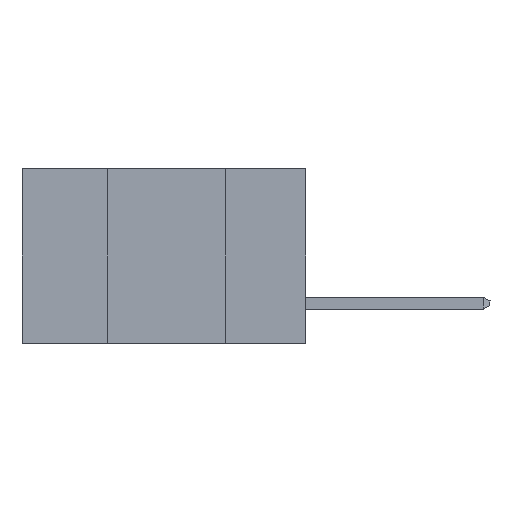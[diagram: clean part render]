
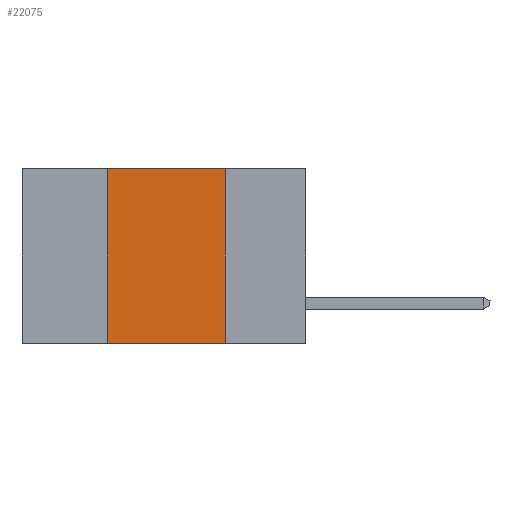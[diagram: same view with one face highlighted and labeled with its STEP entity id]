
A CAD part, left-side view. The second image highlights one B-rep face of the part: STEP entity #22075.
In plain terms, the highlighted planar face has unit normal (-1, 0, 0).
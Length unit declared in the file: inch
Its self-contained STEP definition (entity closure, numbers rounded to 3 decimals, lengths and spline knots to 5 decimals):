
#826 = VECTOR ( 'NONE', #15070, 39.37008 ) ;
#1352 = CARTESIAN_POINT ( 'NONE',  ( 0., 0.42, -0.37 ) ) ;
#1489 = CARTESIAN_POINT ( 'NONE',  ( 0., 0.17, 0. ) ) ;
#1866 = ORIENTED_EDGE ( 'NONE', *, *, #3102, .F. ) ;
#2689 = ORIENTED_EDGE ( 'NONE', *, *, #23865, .F. ) ;
#2981 = FACE_OUTER_BOUND ( 'NONE', #28223, .T. ) ;
#3102 = EDGE_CURVE ( 'NONE', #7601, #16480, #14512, .T. ) ;
#4578 = AXIS2_PLACEMENT_3D ( 'NONE', #21515, #16432, #5238 ) ;
#4989 = ORIENTED_EDGE ( 'NONE', *, *, #14105, .F. ) ;
#5238 = DIRECTION ( 'NONE',  ( 0., 0., -1. ) ) ;
#7601 = VERTEX_POINT ( 'NONE', #1489 ) ;
#12421 = VERTEX_POINT ( 'NONE', #12594 ) ;
#12594 = CARTESIAN_POINT ( 'NONE',  ( 0., 0.42, 0. ) ) ;
#13388 = VECTOR ( 'NONE', #25460, 39.37008 ) ;
#13477 = CARTESIAN_POINT ( 'NONE',  ( 0., 0.17, 0. ) ) ;
#14105 = EDGE_CURVE ( 'NONE', #12421, #7601, #22411, .T. ) ;
#14512 = LINE ( 'NONE', #13477, #13388 ) ;
#14578 = VECTOR ( 'NONE', #15569, 39.37008 ) ;
#14749 = VERTEX_POINT ( 'NONE', #1352 ) ;
#15070 = DIRECTION ( 'NONE',  ( 0., -1., 0. ) ) ;
#15569 = DIRECTION ( 'NONE',  ( 0., -1., 0. ) ) ;
#15824 = CARTESIAN_POINT ( 'NONE',  ( 0., 0.42, 0. ) ) ;
#16432 = DIRECTION ( 'NONE',  ( 1., 0., 0. ) ) ;
#16480 = VERTEX_POINT ( 'NONE', #29526 ) ;
#20097 = CARTESIAN_POINT ( 'NONE',  ( 0., 0.6, -0.37 ) ) ;
#20901 = DIRECTION ( 'NONE',  ( 0., 0., 1. ) ) ;
#21150 = LINE ( 'NONE', #20097, #14578 ) ;
#21515 = CARTESIAN_POINT ( 'NONE',  ( 0., 0.6, 0. ) ) ;
#22075 = ADVANCED_FACE ( 'NONE', ( #2981 ), #25753, .F. ) ;
#22411 = LINE ( 'NONE', #27406, #826 ) ;
#23865 = EDGE_CURVE ( 'NONE', #14749, #12421, #27351, .T. ) ;
#25460 = DIRECTION ( 'NONE',  ( 0., 0., -1. ) ) ;
#25753 = PLANE ( 'NONE',  #4578 ) ;
#26443 = ORIENTED_EDGE ( 'NONE', *, *, #31796, .T. ) ;
#27351 = LINE ( 'NONE', #15824, #30852 ) ;
#27406 = CARTESIAN_POINT ( 'NONE',  ( 0., 0.6, 0. ) ) ;
#28223 = EDGE_LOOP ( 'NONE', ( #1866, #4989, #2689, #26443 ) ) ;
#29526 = CARTESIAN_POINT ( 'NONE',  ( 0., 0.17, -0.37 ) ) ;
#30852 = VECTOR ( 'NONE', #20901, 39.37008 ) ;
#31796 = EDGE_CURVE ( 'NONE', #14749, #16480, #21150, .T. ) ;
